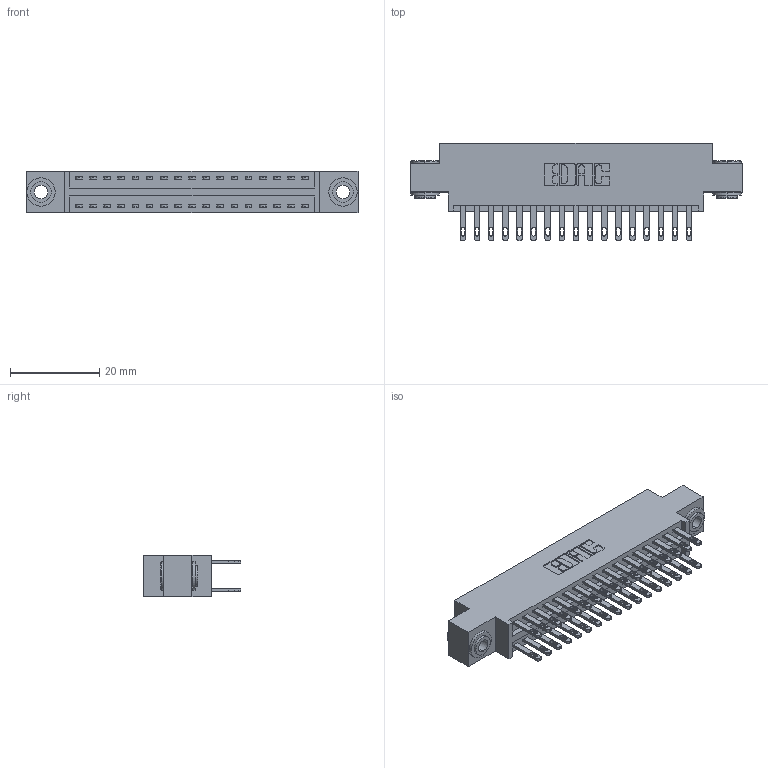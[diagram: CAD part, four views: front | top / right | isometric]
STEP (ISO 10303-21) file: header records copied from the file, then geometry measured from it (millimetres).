
FILE_DESCRIPTION (( 'STEP AP203' ), '1' );
FILE_NAME ('346-034-500-803.STEP', '2022-05-19T19:01:59', ( '' ), ( '' ), 'SwSTEP 2.0', 'SolidWorks 2020', '' );
FILE_SCHEMA (( 'CONFIG_CONTROL_DESIGN' ));
Length unit declared in the file: inch
Products named in the file (4): 345-292-001_345-293-100; 346 Part_0.170 Offset - 0.156 Dia-TH; 346-034-500-803; 345-250-002_345-250-002-102
Assembly tree (37 placements, depth 2):
  346-034-500-803
    346 Part_0.170 Offset - 0.156 Dia-TH
    345-292-001_345-293-100  x34
    345-250-002_345-250-002-102  x2
Bounding box: 74.55 x 21.84 x 9.4 mm (x, y, z)
Volume: 7025.9 mm3; surface area: 10048.8 mm2
Topology: 37 solids, 37 shells, 1810 faces, 5451 edges, 3630 vertices
Faces by surface type: plane 1090, cylinder 712, cone 8
Entity records: 15588 total; most frequent: CARTESIAN_POINT 2585, ORIENTED_EDGE 2510, DIRECTION 2361, EDGE_CURVE 1255, LINE 1027, VECTOR 1027, VERTEX_POINT 834, AXIS2_PLACEMENT_3D 667
